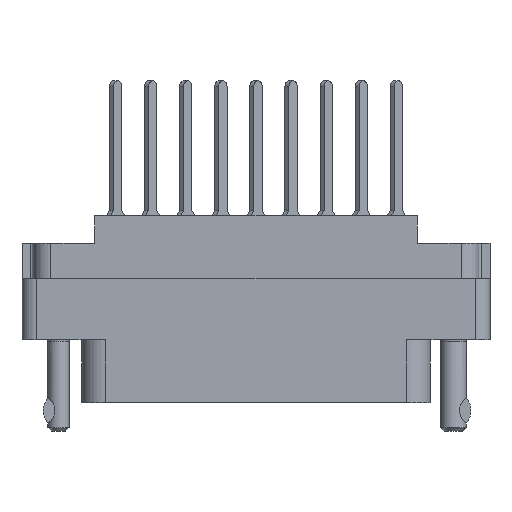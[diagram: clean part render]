
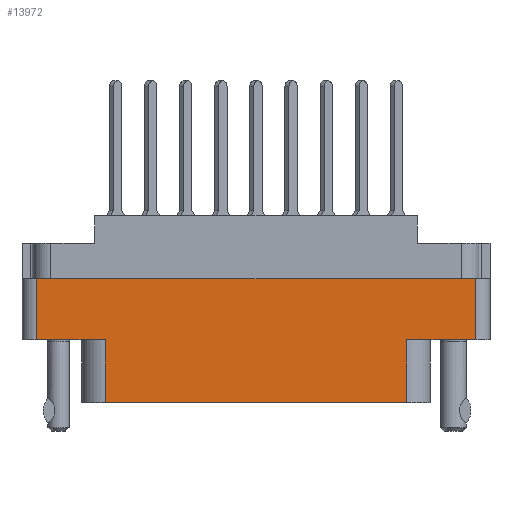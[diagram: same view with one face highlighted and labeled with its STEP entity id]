
A CAD part, front view. The second image highlights one B-rep face of the part: STEP entity #13972.
In plain terms, the highlighted planar face has unit normal (0, -1, 0).
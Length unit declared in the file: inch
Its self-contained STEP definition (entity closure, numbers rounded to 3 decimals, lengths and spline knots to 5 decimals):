
#983 = VECTOR ( 'NONE', #5993, 39.37008 ) ;
#1120 = EDGE_CURVE ( 'NONE', #30902, #43692, #9919, .T. ) ;
#1329 = LINE ( 'NONE', #11687, #38906 ) ;
#2381 = EDGE_CURVE ( 'NONE', #41301, #21361, #32515, .T. ) ;
#3386 = CARTESIAN_POINT ( 'NONE',  ( -0.938, -0.438, -0.798 ) ) ;
#3868 = CARTESIAN_POINT ( 'NONE',  ( 0., -0.438, -0.529 ) ) ;
#3895 = ORIENTED_EDGE ( 'NONE', *, *, #19221, .T. ) ;
#4813 = LINE ( 'NONE', #6602, #983 ) ;
#5512 = VECTOR ( 'NONE', #28588, 39.37008 ) ;
#5748 = DIRECTION ( 'NONE',  ( 1., 0., 0. ) ) ;
#5993 = DIRECTION ( 'NONE',  ( 1., 0., 0. ) ) ;
#6602 = CARTESIAN_POINT ( 'NONE',  ( -1., -0.438, -0.268 ) ) ;
#6922 = DIRECTION ( 'NONE',  ( 0., 0., -1. ) ) ;
#7194 = CARTESIAN_POINT ( 'NONE',  ( -0.938, -0.438, -0.798 ) ) ;
#7787 = CARTESIAN_POINT ( 'NONE',  ( 0.938, -0.438, -0.798 ) ) ;
#8619 = VERTEX_POINT ( 'NONE', #36203 ) ;
#8636 = LINE ( 'NONE', #7787, #44639 ) ;
#8788 = CARTESIAN_POINT ( 'NONE',  ( -0.644, -0.438, -0.798 ) ) ;
#8927 = CARTESIAN_POINT ( 'NONE',  ( 0.644, -0.438, -0.529 ) ) ;
#8958 = CARTESIAN_POINT ( 'NONE',  ( -0.938, -0.438, -0.268 ) ) ;
#9730 = CARTESIAN_POINT ( 'NONE',  ( -0.938, -0.438, -0.798 ) ) ;
#9919 = LINE ( 'NONE', #3868, #5512 ) ;
#10098 = EDGE_CURVE ( 'NONE', #43692, #21361, #1329, .T. ) ;
#10736 = DIRECTION ( 'NONE',  ( 0., 0., 1. ) ) ;
#11687 = CARTESIAN_POINT ( 'NONE',  ( 0.644, -0.438, -0.529 ) ) ;
#12938 = VECTOR ( 'NONE', #35030, 39.37008 ) ;
#13480 = AXIS2_PLACEMENT_3D ( 'NONE', #3386, #28082, #6922 ) ;
#13972 = ADVANCED_FACE ( 'NONE', ( #41431 ), #24528, .T. ) ;
#15339 = ORIENTED_EDGE ( 'NONE', *, *, #36338, .T. ) ;
#15449 = ORIENTED_EDGE ( 'NONE', *, *, #10098, .F. ) ;
#15651 = ORIENTED_EDGE ( 'NONE', *, *, #26622, .F. ) ;
#15890 = ORIENTED_EDGE ( 'NONE', *, *, #1120, .F. ) ;
#18904 = CARTESIAN_POINT ( 'NONE',  ( -0.644, -0.438, -0.529 ) ) ;
#19221 = EDGE_CURVE ( 'NONE', #20968, #41301, #26782, .T. ) ;
#19358 = CARTESIAN_POINT ( 'NONE',  ( 0., -0.438, -0.529 ) ) ;
#19498 = ORIENTED_EDGE ( 'NONE', *, *, #40264, .T. ) ;
#20968 = VERTEX_POINT ( 'NONE', #18904 ) ;
#21361 = VERTEX_POINT ( 'NONE', #42225 ) ;
#21988 = VECTOR ( 'NONE', #5748, 39.37008 ) ;
#24528 = PLANE ( 'NONE',  #13480 ) ;
#24984 = VERTEX_POINT ( 'NONE', #26801 ) ;
#25519 = VERTEX_POINT ( 'NONE', #8958 ) ;
#26622 = EDGE_CURVE ( 'NONE', #24984, #25519, #39314, .T. ) ;
#26782 = LINE ( 'NONE', #31485, #12938 ) ;
#26801 = CARTESIAN_POINT ( 'NONE',  ( -0.938, -0.438, -0.529 ) ) ;
#28082 = DIRECTION ( 'NONE',  ( 0., -1., 0. ) ) ;
#28588 = DIRECTION ( 'NONE',  ( -1., 0., 0. ) ) ;
#30902 = VERTEX_POINT ( 'NONE', #30908 ) ;
#30908 = CARTESIAN_POINT ( 'NONE',  ( 0.938, -0.438, -0.529 ) ) ;
#31485 = CARTESIAN_POINT ( 'NONE',  ( -0.644, -0.438, -0.529 ) ) ;
#32386 = ORIENTED_EDGE ( 'NONE', *, *, #35979, .F. ) ;
#32444 = VECTOR ( 'NONE', #43497, 39.37008 ) ;
#32515 = LINE ( 'NONE', #9730, #21988 ) ;
#35030 = DIRECTION ( 'NONE',  ( 0., 0., -1. ) ) ;
#35979 = EDGE_CURVE ( 'NONE', #25519, #8619, #4813, .T. ) ;
#36203 = CARTESIAN_POINT ( 'NONE',  ( 0.938, -0.438, -0.268 ) ) ;
#36338 = EDGE_CURVE ( 'NONE', #24984, #20968, #42931, .T. ) ;
#38207 = VECTOR ( 'NONE', #39035, 39.37008 ) ;
#38906 = VECTOR ( 'NONE', #39534, 39.37008 ) ;
#39035 = DIRECTION ( 'NONE',  ( 0., 0., 1. ) ) ;
#39314 = LINE ( 'NONE', #7194, #38207 ) ;
#39360 = EDGE_LOOP ( 'NONE', ( #3895, #45692, #15449, #15890, #19498, #32386, #15651, #15339 ) ) ;
#39534 = DIRECTION ( 'NONE',  ( 0., 0., -1. ) ) ;
#40264 = EDGE_CURVE ( 'NONE', #30902, #8619, #8636, .T. ) ;
#41301 = VERTEX_POINT ( 'NONE', #8788 ) ;
#41431 = FACE_OUTER_BOUND ( 'NONE', #39360, .T. ) ;
#42225 = CARTESIAN_POINT ( 'NONE',  ( 0.644, -0.438, -0.798 ) ) ;
#42931 = LINE ( 'NONE', #19358, #32444 ) ;
#43497 = DIRECTION ( 'NONE',  ( 1., 0., 0. ) ) ;
#43692 = VERTEX_POINT ( 'NONE', #8927 ) ;
#44639 = VECTOR ( 'NONE', #10736, 39.37008 ) ;
#45692 = ORIENTED_EDGE ( 'NONE', *, *, #2381, .T. ) ;
